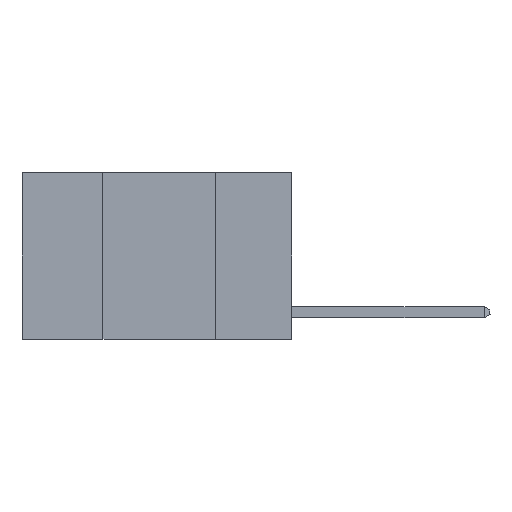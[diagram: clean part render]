
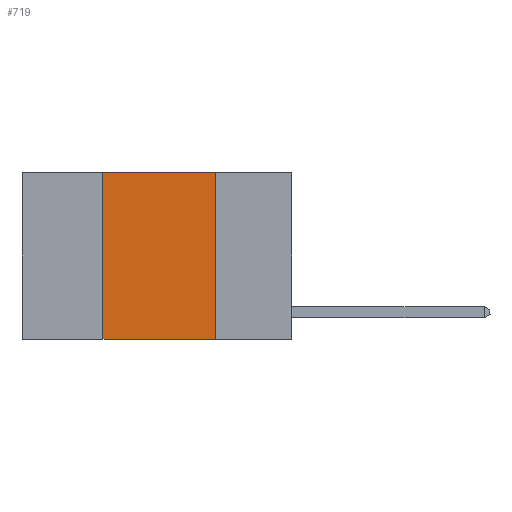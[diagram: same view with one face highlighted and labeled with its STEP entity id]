
A CAD part, left-side view. The second image highlights one B-rep face of the part: STEP entity #719.
In plain terms, the highlighted planar face has unit normal (-1, 0, 0).
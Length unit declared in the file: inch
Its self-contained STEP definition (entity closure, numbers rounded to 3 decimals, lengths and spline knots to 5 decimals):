
#254 = ORIENTED_EDGE ( 'NONE', *, *, #13991, .T. ) ;
#259 = DIRECTION ( 'NONE',  ( 1., 0., 0. ) ) ;
#493 = FACE_OUTER_BOUND ( 'NONE', #12096, .T. ) ;
#708 = EDGE_CURVE ( 'NONE', #10453, #2038, #1628, .T. ) ;
#719 = ADVANCED_FACE ( 'NONE', ( #493 ), #11817, .F. ) ;
#1227 = CARTESIAN_POINT ( 'NONE',  ( 0., 0.17, 0. ) ) ;
#1539 = CARTESIAN_POINT ( 'NONE',  ( 0., 0.42, 0. ) ) ;
#1628 = LINE ( 'NONE', #1539, #10752 ) ;
#2038 = VERTEX_POINT ( 'NONE', #11901 ) ;
#2055 = EDGE_CURVE ( 'NONE', #2038, #5162, #9425, .T. ) ;
#3160 = EDGE_CURVE ( 'NONE', #5162, #7068, #12826, .T. ) ;
#3343 = CARTESIAN_POINT ( 'NONE',  ( 0., 0.42, -0.37 ) ) ;
#5127 = CARTESIAN_POINT ( 'NONE',  ( 0., 0.17, -0.37 ) ) ;
#5162 = VERTEX_POINT ( 'NONE', #9621 ) ;
#5211 = DIRECTION ( 'NONE',  ( 0., 0., -1. ) ) ;
#5932 = ORIENTED_EDGE ( 'NONE', *, *, #2055, .F. ) ;
#6045 = CARTESIAN_POINT ( 'NONE',  ( 0., 0.6, 0. ) ) ;
#6129 = CARTESIAN_POINT ( 'NONE',  ( 0., 0.6, 0. ) ) ;
#6258 = DIRECTION ( 'NONE',  ( 0., 0., 1. ) ) ;
#7068 = VERTEX_POINT ( 'NONE', #5127 ) ;
#7112 = VECTOR ( 'NONE', #10544, 39.37008 ) ;
#7275 = ORIENTED_EDGE ( 'NONE', *, *, #3160, .F. ) ;
#7975 = ORIENTED_EDGE ( 'NONE', *, *, #708, .F. ) ;
#8588 = DIRECTION ( 'NONE',  ( 0., -1., 0. ) ) ;
#9278 = DIRECTION ( 'NONE',  ( 0., 0., -1. ) ) ;
#9425 = LINE ( 'NONE', #6129, #7112 ) ;
#9621 = CARTESIAN_POINT ( 'NONE',  ( 0., 0.17, 0. ) ) ;
#10453 = VERTEX_POINT ( 'NONE', #3343 ) ;
#10544 = DIRECTION ( 'NONE',  ( 0., -1., 0. ) ) ;
#10752 = VECTOR ( 'NONE', #6258, 39.37008 ) ;
#11817 = PLANE ( 'NONE',  #12702 ) ;
#11901 = CARTESIAN_POINT ( 'NONE',  ( 0., 0.42, 0. ) ) ;
#12036 = VECTOR ( 'NONE', #9278, 39.37008 ) ;
#12096 = EDGE_LOOP ( 'NONE', ( #7275, #5932, #7975, #254 ) ) ;
#12483 = VECTOR ( 'NONE', #8588, 39.37008 ) ;
#12702 = AXIS2_PLACEMENT_3D ( 'NONE', #6045, #259, #5211 ) ;
#12826 = LINE ( 'NONE', #1227, #12036 ) ;
#13063 = LINE ( 'NONE', #14532, #12483 ) ;
#13991 = EDGE_CURVE ( 'NONE', #10453, #7068, #13063, .T. ) ;
#14532 = CARTESIAN_POINT ( 'NONE',  ( 0., 0.6, -0.37 ) ) ;
